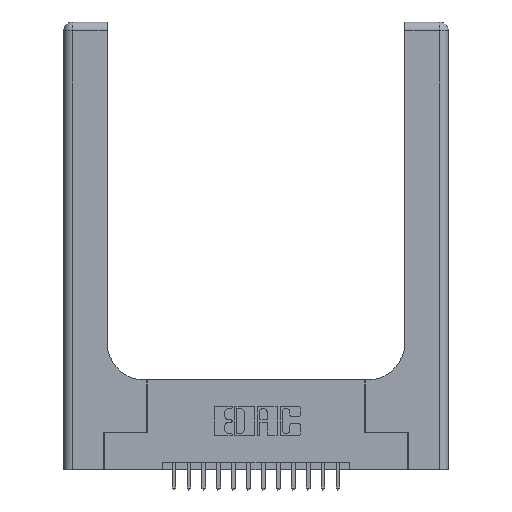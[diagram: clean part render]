
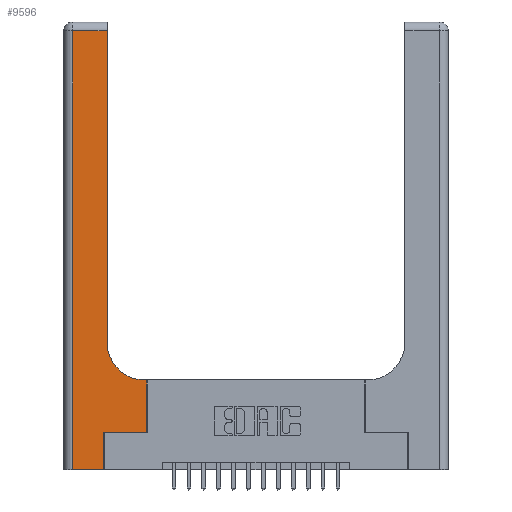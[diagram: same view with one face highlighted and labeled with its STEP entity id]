
A CAD part, top view. The second image highlights one B-rep face of the part: STEP entity #9596.
In plain terms, the highlighted planar face has unit normal (0, 0, 1).
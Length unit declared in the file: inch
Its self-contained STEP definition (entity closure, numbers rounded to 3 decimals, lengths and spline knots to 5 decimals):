
#138 = CARTESIAN_POINT ( 'NONE',  ( 0.2915, 2.94, 0.37 ) ) ;
#823 = DIRECTION ( 'NONE',  ( 1., 0., 0. ) ) ;
#882 = DIRECTION ( 'NONE',  ( 1., 0., 0. ) ) ;
#1087 = EDGE_CURVE ( 'NONE', #10552, #11155, #6910, .T. ) ;
#1281 = CARTESIAN_POINT ( 'NONE',  ( 0.06, 0., 0.37 ) ) ;
#1385 = DIRECTION ( 'NONE',  ( -1., 0., 0. ) ) ;
#1589 = AXIS2_PLACEMENT_3D ( 'NONE', #8015, #6419, #17928 ) ;
#1748 = VERTEX_POINT ( 'NONE', #1281 ) ;
#1957 = CARTESIAN_POINT ( 'NONE',  ( 0.2915, 0.85, 0.37 ) ) ;
#1966 = AXIS2_PLACEMENT_3D ( 'NONE', #9675, #2312, #882 ) ;
#2234 = VECTOR ( 'NONE', #823, 39.37008 ) ;
#2312 = DIRECTION ( 'NONE',  ( 0., 0., -1. ) ) ;
#2374 = CARTESIAN_POINT ( 'NONE',  ( 0.5415, 0.6, 0.37 ) ) ;
#2402 = DIRECTION ( 'NONE',  ( 0., -1., 0. ) ) ;
#2405 = VECTOR ( 'NONE', #16152, 39.37008 ) ;
#2544 = CARTESIAN_POINT ( 'NONE',  ( 0.5585, 0.25, 0.37 ) ) ;
#2674 = CARTESIAN_POINT ( 'NONE',  ( 0.269, 0.25, 0.37 ) ) ;
#3141 = LINE ( 'NONE', #16965, #18289 ) ;
#3146 = EDGE_CURVE ( 'NONE', #10275, #10552, #14909, .T. ) ;
#3758 = DIRECTION ( 'NONE',  ( -1., 0., 0. ) ) ;
#3786 = LINE ( 'NONE', #16191, #15249 ) ;
#3850 = CIRCLE ( 'NONE', #1966, 0.25 ) ;
#3919 = VECTOR ( 'NONE', #4781, 39.37008 ) ;
#4102 = EDGE_LOOP ( 'NONE', ( #8135, #6859, #4155, #13409, #13209, #6221, #17624, #8579, #4797 ) ) ;
#4155 = ORIENTED_EDGE ( 'NONE', *, *, #5627, .T. ) ;
#4176 = CARTESIAN_POINT ( 'NONE',  ( 0., 2.94, 0.37 ) ) ;
#4710 = DIRECTION ( 'NONE',  ( 0., 1., 0. ) ) ;
#4781 = DIRECTION ( 'NONE',  ( 0., 1., 0. ) ) ;
#4797 = ORIENTED_EDGE ( 'NONE', *, *, #9266, .T. ) ;
#4905 = DIRECTION ( 'NONE',  ( 0., 1., 0. ) ) ;
#5130 = CARTESIAN_POINT ( 'NONE',  ( 0.5585, 0.6, 0.37 ) ) ;
#5627 = EDGE_CURVE ( 'NONE', #15817, #1748, #3141, .T. ) ;
#5818 = VERTEX_POINT ( 'NONE', #138 ) ;
#6043 = CARTESIAN_POINT ( 'NONE',  ( 0.269, 0.25, 0.37 ) ) ;
#6221 = ORIENTED_EDGE ( 'NONE', *, *, #10899, .T. ) ;
#6277 = CARTESIAN_POINT ( 'NONE',  ( 0., 0., 0.37 ) ) ;
#6419 = DIRECTION ( 'NONE',  ( 0., 0., -1. ) ) ;
#6833 = VERTEX_POINT ( 'NONE', #1957 ) ;
#6859 = ORIENTED_EDGE ( 'NONE', *, *, #9918, .T. ) ;
#6910 = LINE ( 'NONE', #10831, #8472 ) ;
#7114 = EDGE_CURVE ( 'NONE', #6833, #5818, #10866, .T. ) ;
#8015 = CARTESIAN_POINT ( 'NONE',  ( 0., 3., 0.37 ) ) ;
#8135 = ORIENTED_EDGE ( 'NONE', *, *, #7114, .T. ) ;
#8472 = VECTOR ( 'NONE', #3758, 39.37008 ) ;
#8579 = ORIENTED_EDGE ( 'NONE', *, *, #1087, .T. ) ;
#9159 = EDGE_CURVE ( 'NONE', #1748, #11828, #9680, .T. ) ;
#9266 = EDGE_CURVE ( 'NONE', #11155, #6833, #3850, .T. ) ;
#9367 = CARTESIAN_POINT ( 'NONE',  ( 0.5585, 0.25, 0.37 ) ) ;
#9596 = ADVANCED_FACE ( 'NONE', ( #16688 ), #13452, .F. ) ;
#9675 = CARTESIAN_POINT ( 'NONE',  ( 0.5415, 0.85, 0.37 ) ) ;
#9680 = LINE ( 'NONE', #6277, #2234 ) ;
#9918 = EDGE_CURVE ( 'NONE', #5818, #15817, #16209, .T. ) ;
#10170 = VECTOR ( 'NONE', #4905, 39.37008 ) ;
#10275 = VERTEX_POINT ( 'NONE', #2544 ) ;
#10470 = CARTESIAN_POINT ( 'NONE',  ( 0.2915, 3., 0.37 ) ) ;
#10552 = VERTEX_POINT ( 'NONE', #5130 ) ;
#10831 = CARTESIAN_POINT ( 'NONE',  ( 0.2915, 0.6, 0.37 ) ) ;
#10866 = LINE ( 'NONE', #10470, #3919 ) ;
#10899 = EDGE_CURVE ( 'NONE', #17895, #10275, #14774, .T. ) ;
#11155 = VERTEX_POINT ( 'NONE', #2374 ) ;
#11227 = CARTESIAN_POINT ( 'NONE',  ( 0.269, 0., 0.37 ) ) ;
#11828 = VERTEX_POINT ( 'NONE', #11227 ) ;
#12287 = CARTESIAN_POINT ( 'NONE',  ( 0.06, 2.94, 0.37 ) ) ;
#13209 = ORIENTED_EDGE ( 'NONE', *, *, #17325, .T. ) ;
#13409 = ORIENTED_EDGE ( 'NONE', *, *, #9159, .T. ) ;
#13452 = PLANE ( 'NONE',  #1589 ) ;
#13914 = VECTOR ( 'NONE', #1385, 39.37008 ) ;
#14774 = LINE ( 'NONE', #6043, #2405 ) ;
#14909 = LINE ( 'NONE', #9367, #10170 ) ;
#15249 = VECTOR ( 'NONE', #4710, 39.37008 ) ;
#15817 = VERTEX_POINT ( 'NONE', #12287 ) ;
#16152 = DIRECTION ( 'NONE',  ( 1., 0., 0. ) ) ;
#16191 = CARTESIAN_POINT ( 'NONE',  ( 0.269, 0., 0.37 ) ) ;
#16209 = LINE ( 'NONE', #4176, #13914 ) ;
#16688 = FACE_OUTER_BOUND ( 'NONE', #4102, .T. ) ;
#16965 = CARTESIAN_POINT ( 'NONE',  ( 0.06, 3., 0.37 ) ) ;
#17325 = EDGE_CURVE ( 'NONE', #11828, #17895, #3786, .T. ) ;
#17624 = ORIENTED_EDGE ( 'NONE', *, *, #3146, .T. ) ;
#17895 = VERTEX_POINT ( 'NONE', #2674 ) ;
#17928 = DIRECTION ( 'NONE',  ( -1., 0., 0. ) ) ;
#18289 = VECTOR ( 'NONE', #2402, 39.37008 ) ;
